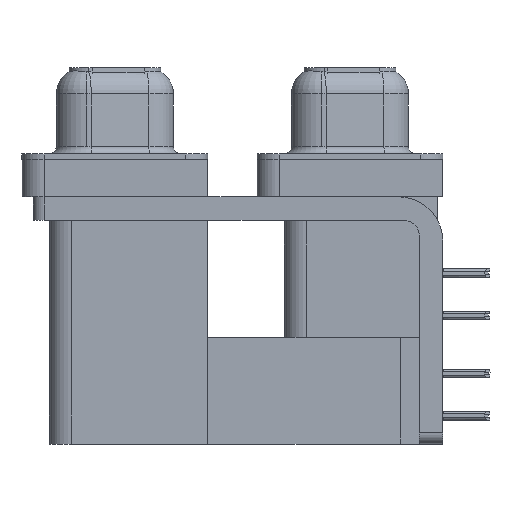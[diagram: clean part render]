
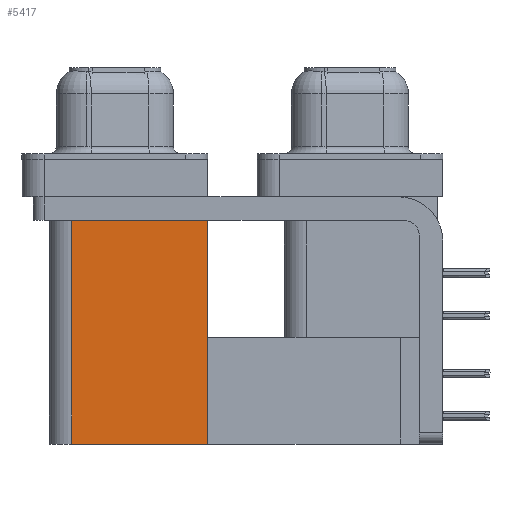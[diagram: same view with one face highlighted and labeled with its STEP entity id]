
A CAD part, left-side view. The second image highlights one B-rep face of the part: STEP entity #5417.
In plain terms, the highlighted planar face has unit normal (-1, 0, 0).
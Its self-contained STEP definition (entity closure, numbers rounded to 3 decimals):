
#1403 = ORIENTED_EDGE ( 'NONE', *, *, #30801, .F. ) ;
#2016 = CARTESIAN_POINT ( 'NONE',  ( 3.765, 9.6, -2.5 ) ) ;
#3694 = VERTEX_POINT ( 'NONE', #18796 ) ;
#4561 = ORIENTED_EDGE ( 'NONE', *, *, #17156, .F. ) ;
#4914 = ORIENTED_EDGE ( 'NONE', *, *, #39063, .T. ) ;
#5081 = EDGE_LOOP ( 'NONE', ( #4914, #1403, #4561, #34799 ) ) ;
#5096 = CARTESIAN_POINT ( 'NONE',  ( 3.765, 9.6, -19.2 ) ) ;
#5417 = ADVANCED_FACE ( 'NONE', ( #44672 ), #44197, .F. ) ;
#6292 = VECTOR ( 'NONE', #29824, 1000. ) ;
#11425 = EDGE_CURVE ( 'NONE', #22850, #28512, #38152, .T. ) ;
#12738 = LINE ( 'NONE', #5096, #47149 ) ;
#13769 = VECTOR ( 'NONE', #48506, 1000. ) ;
#15482 = CARTESIAN_POINT ( 'NONE',  ( 3.765, 9.6, -19.2 ) ) ;
#15739 = CARTESIAN_POINT ( 'NONE',  ( 3.765, 9.6, -2.5 ) ) ;
#16165 = DIRECTION ( 'NONE',  ( 0., 1., 0. ) ) ;
#17156 = EDGE_CURVE ( 'NONE', #22850, #3694, #12738, .T. ) ;
#17765 = DIRECTION ( 'NONE',  ( 1., 0., 0. ) ) ;
#18796 = CARTESIAN_POINT ( 'NONE',  ( 3.765, 18.8, -19.2 ) ) ;
#22161 = VECTOR ( 'NONE', #37917, 1000. ) ;
#22675 = LINE ( 'NONE', #15739, #6292 ) ;
#22850 = VERTEX_POINT ( 'NONE', #15482 ) ;
#25414 = CARTESIAN_POINT ( 'NONE',  ( 3.765, 9.6, -19.2 ) ) ;
#28512 = VERTEX_POINT ( 'NONE', #2016 ) ;
#28864 = DIRECTION ( 'NONE',  ( 0., 0., -1. ) ) ;
#29824 = DIRECTION ( 'NONE',  ( 0., 1., 0. ) ) ;
#30801 = EDGE_CURVE ( 'NONE', #3694, #45762, #37408, .T. ) ;
#34799 = ORIENTED_EDGE ( 'NONE', *, *, #11425, .T. ) ;
#37408 = LINE ( 'NONE', #45314, #13769 ) ;
#37917 = DIRECTION ( 'NONE',  ( 0., 0., 1. ) ) ;
#38123 = CARTESIAN_POINT ( 'NONE',  ( 3.765, 18.8, -2.5 ) ) ;
#38152 = LINE ( 'NONE', #45075, #22161 ) ;
#39063 = EDGE_CURVE ( 'NONE', #28512, #45762, #22675, .T. ) ;
#44197 = PLANE ( 'NONE',  #45199 ) ;
#44672 = FACE_OUTER_BOUND ( 'NONE', #5081, .T. ) ;
#45075 = CARTESIAN_POINT ( 'NONE',  ( 3.765, 9.6, -19.2 ) ) ;
#45199 = AXIS2_PLACEMENT_3D ( 'NONE', #25414, #17765, #28864 ) ;
#45314 = CARTESIAN_POINT ( 'NONE',  ( 3.765, 18.8, -19.2 ) ) ;
#45762 = VERTEX_POINT ( 'NONE', #38123 ) ;
#47149 = VECTOR ( 'NONE', #16165, 1000. ) ;
#48506 = DIRECTION ( 'NONE',  ( 0., 0., 1. ) ) ;
